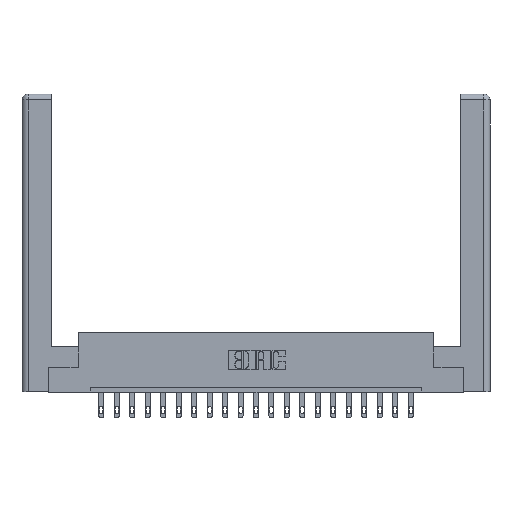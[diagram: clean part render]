
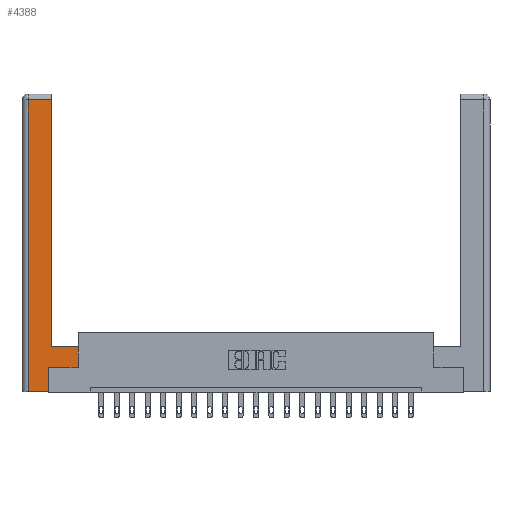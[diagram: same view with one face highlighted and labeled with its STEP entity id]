
A CAD part, top view. The second image highlights one B-rep face of the part: STEP entity #4388.
In plain terms, the highlighted planar face has unit normal (0, 0, 1).
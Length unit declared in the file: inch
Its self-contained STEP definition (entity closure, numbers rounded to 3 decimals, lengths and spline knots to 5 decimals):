
#738 = VERTEX_POINT ( 'NONE', #9879 ) ;
#862 = EDGE_CURVE ( 'NONE', #11812, #2437, #18951, .T. ) ;
#1525 = PLANE ( 'NONE',  #19847 ) ;
#1583 = ORIENTED_EDGE ( 'NONE', *, *, #862, .T. ) ;
#1869 = VERTEX_POINT ( 'NONE', #17478 ) ;
#2334 = CARTESIAN_POINT ( 'NONE',  ( 0.565, 0.245, 0. ) ) ;
#2336 = ORIENTED_EDGE ( 'NONE', *, *, #5249, .T. ) ;
#2437 = VERTEX_POINT ( 'NONE', #3516 ) ;
#2639 = DIRECTION ( 'NONE',  ( 0., 1., 0. ) ) ;
#2704 = VERTEX_POINT ( 'NONE', #5095 ) ;
#2854 = VECTOR ( 'NONE', #2639, 39.37008 ) ;
#3106 = DIRECTION ( 'NONE',  ( 0., 1., 0. ) ) ;
#3516 = CARTESIAN_POINT ( 'NONE',  ( 0.295, 0.45, 0. ) ) ;
#3547 = CARTESIAN_POINT ( 'NONE',  ( 0.0615, 0., 0. ) ) ;
#3867 = EDGE_CURVE ( 'NONE', #18124, #11812, #10509, .T. ) ;
#4132 = CARTESIAN_POINT ( 'NONE',  ( 0.265, 0.245, 0. ) ) ;
#4388 = ADVANCED_FACE ( 'NONE', ( #7201 ), #1525, .F. ) ;
#4772 = DIRECTION ( 'NONE',  ( 0., 1., 0. ) ) ;
#5095 = CARTESIAN_POINT ( 'NONE',  ( 0.0615, 2.94, 0. ) ) ;
#5133 = VECTOR ( 'NONE', #17955, 39.37008 ) ;
#5200 = VECTOR ( 'NONE', #4772, 39.37008 ) ;
#5249 = EDGE_CURVE ( 'NONE', #2704, #1869, #5654, .T. ) ;
#5654 = LINE ( 'NONE', #3547, #5133 ) ;
#6169 = ORIENTED_EDGE ( 'NONE', *, *, #14032, .T. ) ;
#6229 = VECTOR ( 'NONE', #3106, 39.37008 ) ;
#6436 = CARTESIAN_POINT ( 'NONE',  ( 0., 0., 0. ) ) ;
#6677 = ORIENTED_EDGE ( 'NONE', *, *, #19533, .T. ) ;
#6879 = EDGE_LOOP ( 'NONE', ( #18737, #10905, #2336, #6169, #12984, #6677, #19500, #1583 ) ) ;
#7201 = FACE_OUTER_BOUND ( 'NONE', #6879, .T. ) ;
#7827 = CARTESIAN_POINT ( 'NONE',  ( 0.265, 0.245, 0. ) ) ;
#8146 = DIRECTION ( 'NONE',  ( 1., 0., 0. ) ) ;
#8600 = VECTOR ( 'NONE', #17866, 39.37008 ) ;
#9240 = EDGE_CURVE ( 'NONE', #13428, #11112, #20775, .T. ) ;
#9879 = CARTESIAN_POINT ( 'NONE',  ( 0.295, 2.94, 0. ) ) ;
#10011 = CARTESIAN_POINT ( 'NONE',  ( 0.295, 3., 0. ) ) ;
#10246 = EDGE_CURVE ( 'NONE', #738, #2704, #11187, .T. ) ;
#10509 = LINE ( 'NONE', #15907, #6229 ) ;
#10836 = DIRECTION ( 'NONE',  ( 1., 0., 0. ) ) ;
#10905 = ORIENTED_EDGE ( 'NONE', *, *, #10246, .T. ) ;
#11112 = VERTEX_POINT ( 'NONE', #7827 ) ;
#11167 = VECTOR ( 'NONE', #19017, 39.37008 ) ;
#11187 = LINE ( 'NONE', #19978, #8600 ) ;
#11436 = CARTESIAN_POINT ( 'NONE',  ( 0.565, 0.245, 0. ) ) ;
#11812 = VERTEX_POINT ( 'NONE', #14919 ) ;
#12984 = ORIENTED_EDGE ( 'NONE', *, *, #9240, .T. ) ;
#13428 = VERTEX_POINT ( 'NONE', #17179 ) ;
#13801 = LINE ( 'NONE', #10011, #5200 ) ;
#13865 = VECTOR ( 'NONE', #8146, 39.37008 ) ;
#14032 = EDGE_CURVE ( 'NONE', #1869, #13428, #14308, .T. ) ;
#14308 = LINE ( 'NONE', #15465, #18053 ) ;
#14919 = CARTESIAN_POINT ( 'NONE',  ( 0.565, 0.45, 0. ) ) ;
#15465 = CARTESIAN_POINT ( 'NONE',  ( 0.265, 0., 0. ) ) ;
#15907 = CARTESIAN_POINT ( 'NONE',  ( 0.565, 0.45, 0. ) ) ;
#16021 = DIRECTION ( 'NONE',  ( 0., 0., -1. ) ) ;
#17175 = EDGE_CURVE ( 'NONE', #2437, #738, #13801, .T. ) ;
#17179 = CARTESIAN_POINT ( 'NONE',  ( 0.265, 0., 0. ) ) ;
#17478 = CARTESIAN_POINT ( 'NONE',  ( 0.0615, 0., 0. ) ) ;
#17505 = DIRECTION ( 'NONE',  ( -1., 0., 0. ) ) ;
#17866 = DIRECTION ( 'NONE',  ( -1., 0., 0. ) ) ;
#17955 = DIRECTION ( 'NONE',  ( 0., -1., 0. ) ) ;
#18053 = VECTOR ( 'NONE', #10836, 39.37008 ) ;
#18124 = VERTEX_POINT ( 'NONE', #2334 ) ;
#18737 = ORIENTED_EDGE ( 'NONE', *, *, #17175, .T. ) ;
#18951 = LINE ( 'NONE', #19080, #11167 ) ;
#19017 = DIRECTION ( 'NONE',  ( -1., 0., 0. ) ) ;
#19080 = CARTESIAN_POINT ( 'NONE',  ( 0.295, 0.45, 0. ) ) ;
#19500 = ORIENTED_EDGE ( 'NONE', *, *, #3867, .T. ) ;
#19533 = EDGE_CURVE ( 'NONE', #11112, #18124, #20671, .T. ) ;
#19847 = AXIS2_PLACEMENT_3D ( 'NONE', #6436, #16021, #17505 ) ;
#19978 = CARTESIAN_POINT ( 'NONE',  ( 0.0615, 2.94, 0. ) ) ;
#20671 = LINE ( 'NONE', #11436, #13865 ) ;
#20775 = LINE ( 'NONE', #4132, #2854 ) ;
